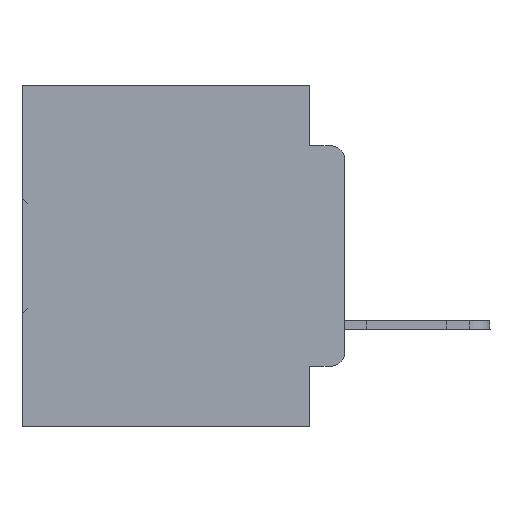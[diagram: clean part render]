
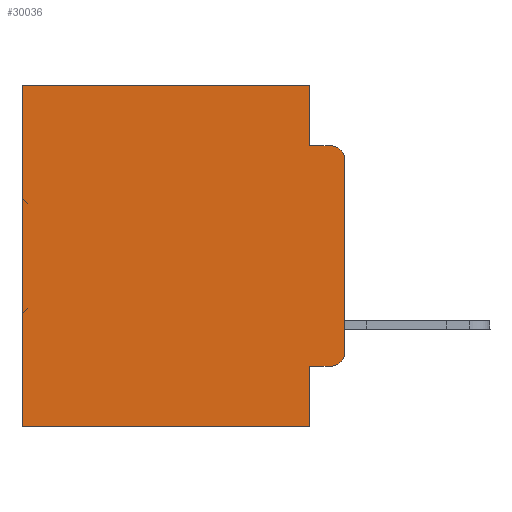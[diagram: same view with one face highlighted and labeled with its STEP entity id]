
A CAD part, left-side view. The second image highlights one B-rep face of the part: STEP entity #30036.
In plain terms, the highlighted planar face has unit normal (-1, 0, 0).
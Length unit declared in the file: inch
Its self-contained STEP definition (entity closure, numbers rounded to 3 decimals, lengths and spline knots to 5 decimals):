
#105 = VERTEX_POINT ( 'NONE', #2929 ) ;
#481 = ORIENTED_EDGE ( 'NONE', *, *, #2140, .T. ) ;
#507 = VECTOR ( 'NONE', #14457, 39.37008 ) ;
#1106 = ORIENTED_EDGE ( 'NONE', *, *, #12339, .T. ) ;
#1178 = DIRECTION ( 'NONE',  ( 0., 0., -1. ) ) ;
#1785 = CARTESIAN_POINT ( 'NONE',  ( 0.298, 0.473, 0. ) ) ;
#1789 = ORIENTED_EDGE ( 'NONE', *, *, #9679, .F. ) ;
#2140 = EDGE_CURVE ( 'NONE', #36015, #28152, #2659, .T. ) ;
#2596 = CARTESIAN_POINT ( 'NONE',  ( 0.298, 0., -0.5 ) ) ;
#2659 = LINE ( 'NONE', #8486, #23269 ) ;
#2791 = CIRCLE ( 'NONE', #27408, 0.02 ) ;
#2809 = CARTESIAN_POINT ( 'NONE',  ( 0.298, 0., 0. ) ) ;
#2929 = CARTESIAN_POINT ( 'NONE',  ( 0.298, 0.051, -0.5 ) ) ;
#2972 = VERTEX_POINT ( 'NONE', #5387 ) ;
#3990 = FACE_OUTER_BOUND ( 'NONE', #4625, .T. ) ;
#4114 = DIRECTION ( 'NONE',  ( 0., 0., -1. ) ) ;
#4595 = CARTESIAN_POINT ( 'NONE',  ( 0.298, 0.051, -0.4115 ) ) ;
#4625 = EDGE_LOOP ( 'NONE', ( #21906, #11024, #34386, #9222, #19245, #481, #6004, #1789, #1106, #29653 ) ) ;
#4807 = DIRECTION ( 'NONE',  ( 0., 0., -1. ) ) ;
#5198 = CARTESIAN_POINT ( 'NONE',  ( 0.298, 0.473, -0.5 ) ) ;
#5387 = CARTESIAN_POINT ( 'NONE',  ( 0.298, 0., -0.3915 ) ) ;
#5644 = DIRECTION ( 'NONE',  ( 0., 0., -1. ) ) ;
#5986 = CARTESIAN_POINT ( 'NONE',  ( 0.298, 0.02, -0.4115 ) ) ;
#6004 = ORIENTED_EDGE ( 'NONE', *, *, #19476, .F. ) ;
#6337 = AXIS2_PLACEMENT_3D ( 'NONE', #34327, #25457, #13952 ) ;
#6665 = EDGE_CURVE ( 'NONE', #16641, #19720, #29533, .T. ) ;
#8257 = LINE ( 'NONE', #2809, #507 ) ;
#8486 = CARTESIAN_POINT ( 'NONE',  ( 0.298, 0.473, 0. ) ) ;
#8622 = DIRECTION ( 'NONE',  ( 0., 0., -1. ) ) ;
#9222 = ORIENTED_EDGE ( 'NONE', *, *, #6665, .F. ) ;
#9679 = EDGE_CURVE ( 'NONE', #29705, #105, #18414, .T. ) ;
#10368 = CARTESIAN_POINT ( 'NONE',  ( 0.298, 0.051, -0.0885 ) ) ;
#10545 = AXIS2_PLACEMENT_3D ( 'NONE', #26961, #17573, #1178 ) ;
#11024 = ORIENTED_EDGE ( 'NONE', *, *, #22246, .T. ) ;
#12203 = CARTESIAN_POINT ( 'NONE',  ( 0.298, 0.051, 0. ) ) ;
#12339 = EDGE_CURVE ( 'NONE', #29705, #16677, #12448, .T. ) ;
#12448 = LINE ( 'NONE', #23961, #16471 ) ;
#12564 = VECTOR ( 'NONE', #8622, 39.37008 ) ;
#13679 = DIRECTION ( 'NONE',  ( 0., 1., 0. ) ) ;
#13692 = VECTOR ( 'NONE', #4807, 39.37008 ) ;
#13952 = DIRECTION ( 'NONE',  ( 0., 0., -1. ) ) ;
#14457 = DIRECTION ( 'NONE',  ( 0., 1., 0. ) ) ;
#15474 = PLANE ( 'NONE',  #10545 ) ;
#16093 = CARTESIAN_POINT ( 'NONE',  ( 0.298, 0.051, -0.0885 ) ) ;
#16471 = VECTOR ( 'NONE', #29763, 39.37008 ) ;
#16641 = VERTEX_POINT ( 'NONE', #32669 ) ;
#16677 = VERTEX_POINT ( 'NONE', #5986 ) ;
#17573 = DIRECTION ( 'NONE',  ( 1., 0., 0. ) ) ;
#17790 = CIRCLE ( 'NONE', #6337, 0.02 ) ;
#18414 = LINE ( 'NONE', #29890, #20506 ) ;
#19245 = ORIENTED_EDGE ( 'NONE', *, *, #26162, .T. ) ;
#19476 = EDGE_CURVE ( 'NONE', #105, #28152, #22930, .T. ) ;
#19720 = VERTEX_POINT ( 'NONE', #16093 ) ;
#19921 = LINE ( 'NONE', #22953, #12564 ) ;
#20506 = VECTOR ( 'NONE', #4114, 39.37008 ) ;
#21864 = DIRECTION ( 'NONE',  ( 0., -1., 0. ) ) ;
#21906 = ORIENTED_EDGE ( 'NONE', *, *, #35392, .F. ) ;
#22246 = EDGE_CURVE ( 'NONE', #29215, #31692, #2791, .T. ) ;
#22930 = LINE ( 'NONE', #2596, #24842 ) ;
#22953 = CARTESIAN_POINT ( 'NONE',  ( 0.298, 0., 0. ) ) ;
#23269 = VECTOR ( 'NONE', #5644, 39.37008 ) ;
#23574 = CARTESIAN_POINT ( 'NONE',  ( 0.298, 0.02, -0.0885 ) ) ;
#23961 = CARTESIAN_POINT ( 'NONE',  ( 0.298, 0.051, -0.4115 ) ) ;
#24640 = EDGE_CURVE ( 'NONE', #19720, #31692, #24696, .T. ) ;
#24696 = LINE ( 'NONE', #10368, #37140 ) ;
#24842 = VECTOR ( 'NONE', #13679, 39.37008 ) ;
#25457 = DIRECTION ( 'NONE',  ( -1., 0., 0. ) ) ;
#26162 = EDGE_CURVE ( 'NONE', #16641, #36015, #8257, .T. ) ;
#26961 = CARTESIAN_POINT ( 'NONE',  ( 0.298, 0., 0. ) ) ;
#27098 = CARTESIAN_POINT ( 'NONE',  ( 0.298, 0., -0.1085 ) ) ;
#27408 = AXIS2_PLACEMENT_3D ( 'NONE', #28126, #37019, #36647 ) ;
#28126 = CARTESIAN_POINT ( 'NONE',  ( 0.298, 0.02, -0.1085 ) ) ;
#28152 = VERTEX_POINT ( 'NONE', #5198 ) ;
#29215 = VERTEX_POINT ( 'NONE', #27098 ) ;
#29533 = LINE ( 'NONE', #12203, #13692 ) ;
#29653 = ORIENTED_EDGE ( 'NONE', *, *, #30233, .T. ) ;
#29705 = VERTEX_POINT ( 'NONE', #4595 ) ;
#29763 = DIRECTION ( 'NONE',  ( 0., -1., 0. ) ) ;
#29890 = CARTESIAN_POINT ( 'NONE',  ( 0.298, 0.051, 0. ) ) ;
#30036 = ADVANCED_FACE ( 'NONE', ( #3990 ), #15474, .F. ) ;
#30233 = EDGE_CURVE ( 'NONE', #16677, #2972, #17790, .T. ) ;
#31692 = VERTEX_POINT ( 'NONE', #23574 ) ;
#32669 = CARTESIAN_POINT ( 'NONE',  ( 0.298, 0.051, 0. ) ) ;
#34327 = CARTESIAN_POINT ( 'NONE',  ( 0.298, 0.02, -0.3915 ) ) ;
#34386 = ORIENTED_EDGE ( 'NONE', *, *, #24640, .F. ) ;
#35392 = EDGE_CURVE ( 'NONE', #29215, #2972, #19921, .T. ) ;
#36015 = VERTEX_POINT ( 'NONE', #1785 ) ;
#36647 = DIRECTION ( 'NONE',  ( 0., 0., -1. ) ) ;
#37019 = DIRECTION ( 'NONE',  ( -1., 0., 0. ) ) ;
#37140 = VECTOR ( 'NONE', #21864, 39.37008 ) ;
